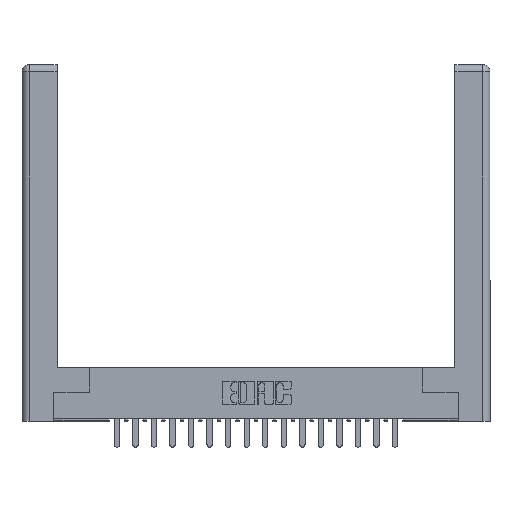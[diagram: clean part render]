
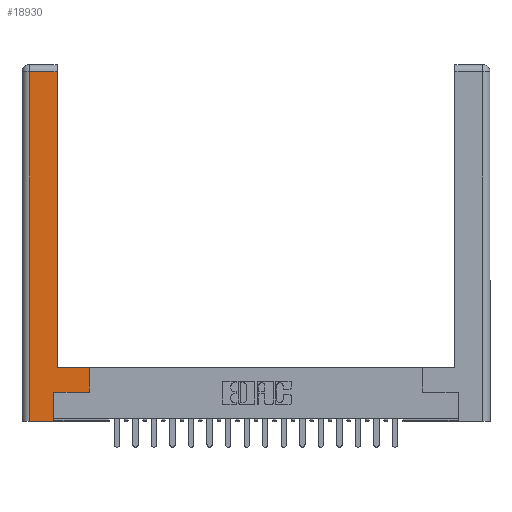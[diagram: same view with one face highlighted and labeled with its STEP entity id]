
A CAD part, top view. The second image highlights one B-rep face of the part: STEP entity #18930.
In plain terms, the highlighted planar face has unit normal (0, 0, 1).
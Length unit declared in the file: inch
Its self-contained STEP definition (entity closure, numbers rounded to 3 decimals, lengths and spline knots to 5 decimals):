
#444 = LINE ( 'NONE', #12679, #22957 ) ;
#637 = EDGE_CURVE ( 'NONE', #10409, #14538, #22021, .T. ) ;
#874 = EDGE_CURVE ( 'NONE', #14538, #22932, #12819, .T. ) ;
#1270 = DIRECTION ( 'NONE',  ( -1., 0., 0. ) ) ;
#1806 = CARTESIAN_POINT ( 'NONE',  ( 0.265, 0.245, 0. ) ) ;
#1875 = DIRECTION ( 'NONE',  ( 0., 0., -1. ) ) ;
#2071 = DIRECTION ( 'NONE',  ( 1., 0., 0. ) ) ;
#2633 = CARTESIAN_POINT ( 'NONE',  ( 0.0615, 2.94, 0. ) ) ;
#3732 = DIRECTION ( 'NONE',  ( 0., 1., 0. ) ) ;
#3847 = VECTOR ( 'NONE', #12418, 39.37008 ) ;
#4085 = ORIENTED_EDGE ( 'NONE', *, *, #18276, .T. ) ;
#4600 = VERTEX_POINT ( 'NONE', #11866 ) ;
#4943 = CARTESIAN_POINT ( 'NONE',  ( 0.295, 0.45, 0. ) ) ;
#5035 = VECTOR ( 'NONE', #3732, 39.37008 ) ;
#5285 = CARTESIAN_POINT ( 'NONE',  ( 0.565, 0.245, 0. ) ) ;
#6479 = CARTESIAN_POINT ( 'NONE',  ( 0.565, 0.45, 0. ) ) ;
#6622 = CARTESIAN_POINT ( 'NONE',  ( 0.0615, 0., 0. ) ) ;
#7503 = LINE ( 'NONE', #11610, #17548 ) ;
#7781 = ORIENTED_EDGE ( 'NONE', *, *, #11224, .T. ) ;
#8106 = VECTOR ( 'NONE', #11820, 39.37008 ) ;
#8262 = LINE ( 'NONE', #5285, #3847 ) ;
#8598 = CARTESIAN_POINT ( 'NONE',  ( 0.0615, 0., 0. ) ) ;
#9560 = ORIENTED_EDGE ( 'NONE', *, *, #17725, .T. ) ;
#10003 = VECTOR ( 'NONE', #22827, 39.37008 ) ;
#10334 = EDGE_CURVE ( 'NONE', #4600, #11550, #7503, .T. ) ;
#10409 = VERTEX_POINT ( 'NONE', #19221 ) ;
#10887 = PLANE ( 'NONE',  #21611 ) ;
#11124 = ORIENTED_EDGE ( 'NONE', *, *, #874, .T. ) ;
#11224 = EDGE_CURVE ( 'NONE', #15602, #17481, #8262, .T. ) ;
#11550 = VERTEX_POINT ( 'NONE', #4943 ) ;
#11610 = CARTESIAN_POINT ( 'NONE',  ( 0.295, 0.45, 0. ) ) ;
#11667 = LINE ( 'NONE', #1806, #5035 ) ;
#11820 = DIRECTION ( 'NONE',  ( 0., 1., 0. ) ) ;
#11866 = CARTESIAN_POINT ( 'NONE',  ( 0.565, 0.45, 0. ) ) ;
#12418 = DIRECTION ( 'NONE',  ( 1., 0., 0. ) ) ;
#12679 = CARTESIAN_POINT ( 'NONE',  ( 0.265, 0., 0. ) ) ;
#12819 = LINE ( 'NONE', #6622, #10003 ) ;
#12901 = VECTOR ( 'NONE', #21312, 39.37008 ) ;
#12958 = ORIENTED_EDGE ( 'NONE', *, *, #10334, .T. ) ;
#13043 = DIRECTION ( 'NONE',  ( -1., 0., 0. ) ) ;
#14538 = VERTEX_POINT ( 'NONE', #21133 ) ;
#14542 = ORIENTED_EDGE ( 'NONE', *, *, #16657, .T. ) ;
#14914 = CARTESIAN_POINT ( 'NONE',  ( 0.265, 0.245, 0. ) ) ;
#15091 = LINE ( 'NONE', #6479, #8106 ) ;
#15262 = CARTESIAN_POINT ( 'NONE',  ( 0.265, 0., 0. ) ) ;
#15602 = VERTEX_POINT ( 'NONE', #14914 ) ;
#15604 = EDGE_LOOP ( 'NONE', ( #14542, #16001, #11124, #20523, #4085, #7781, #9560, #12958 ) ) ;
#15912 = VECTOR ( 'NONE', #13043, 39.37008 ) ;
#16001 = ORIENTED_EDGE ( 'NONE', *, *, #637, .T. ) ;
#16657 = EDGE_CURVE ( 'NONE', #11550, #10409, #18501, .T. ) ;
#16894 = EDGE_CURVE ( 'NONE', #22932, #18165, #444, .T. ) ;
#17481 = VERTEX_POINT ( 'NONE', #18281 ) ;
#17548 = VECTOR ( 'NONE', #1270, 39.37008 ) ;
#17725 = EDGE_CURVE ( 'NONE', #17481, #4600, #15091, .T. ) ;
#18165 = VERTEX_POINT ( 'NONE', #15262 ) ;
#18182 = CARTESIAN_POINT ( 'NONE',  ( 0., 0., 0. ) ) ;
#18276 = EDGE_CURVE ( 'NONE', #18165, #15602, #11667, .T. ) ;
#18281 = CARTESIAN_POINT ( 'NONE',  ( 0.565, 0.245, 0. ) ) ;
#18501 = LINE ( 'NONE', #21236, #12901 ) ;
#18930 = ADVANCED_FACE ( 'NONE', ( #19214 ), #10887, .F. ) ;
#19214 = FACE_OUTER_BOUND ( 'NONE', #15604, .T. ) ;
#19221 = CARTESIAN_POINT ( 'NONE',  ( 0.295, 2.94, 0. ) ) ;
#20523 = ORIENTED_EDGE ( 'NONE', *, *, #16894, .T. ) ;
#21133 = CARTESIAN_POINT ( 'NONE',  ( 0.0615, 2.94, 0. ) ) ;
#21236 = CARTESIAN_POINT ( 'NONE',  ( 0.295, 3., 0. ) ) ;
#21312 = DIRECTION ( 'NONE',  ( 0., 1., 0. ) ) ;
#21586 = DIRECTION ( 'NONE',  ( -1., 0., 0. ) ) ;
#21611 = AXIS2_PLACEMENT_3D ( 'NONE', #18182, #1875, #21586 ) ;
#22021 = LINE ( 'NONE', #2633, #15912 ) ;
#22827 = DIRECTION ( 'NONE',  ( 0., -1., 0. ) ) ;
#22932 = VERTEX_POINT ( 'NONE', #8598 ) ;
#22957 = VECTOR ( 'NONE', #2071, 39.37008 ) ;
